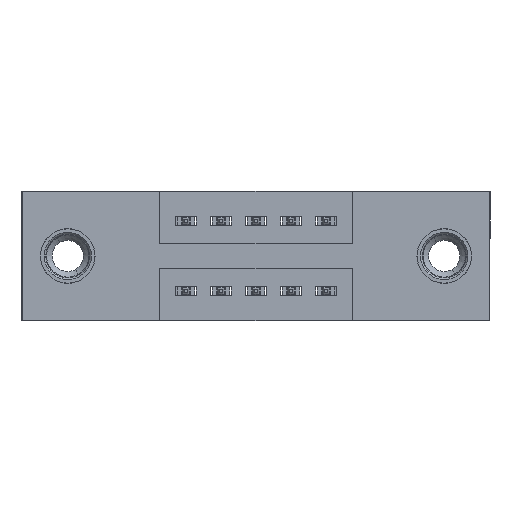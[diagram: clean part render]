
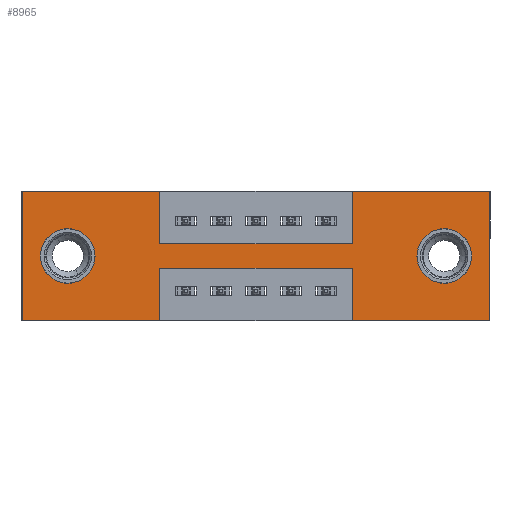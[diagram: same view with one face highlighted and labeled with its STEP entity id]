
A CAD part, front view. The second image highlights one B-rep face of the part: STEP entity #8965.
In plain terms, the highlighted planar face has unit normal (0, -1, 0).
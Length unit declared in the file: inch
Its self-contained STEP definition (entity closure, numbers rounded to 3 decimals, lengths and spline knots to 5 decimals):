
#48 = AXIS2_PLACEMENT_3D ( 'NONE', #10438, #9394, #13650 ) ;
#277 = CARTESIAN_POINT ( 'NONE',  ( 0.3925, 0., -0.15 ) ) ;
#557 = VERTEX_POINT ( 'NONE', #3765 ) ;
#641 = CARTESIAN_POINT ( 'NONE',  ( 0.3925, 0., 0. ) ) ;
#711 = VECTOR ( 'NONE', #12279, 39.37008 ) ;
#821 = EDGE_CURVE ( 'NONE', #13624, #557, #13502, .T. ) ;
#884 = DIRECTION ( 'NONE',  ( 0., 0., 1. ) ) ;
#1006 = CARTESIAN_POINT ( 'NONE',  ( 0.9425, 0., -0.15 ) ) ;
#1064 = VERTEX_POINT ( 'NONE', #1105 ) ;
#1100 = ORIENTED_EDGE ( 'NONE', *, *, #4428, .T. ) ;
#1105 = CARTESIAN_POINT ( 'NONE',  ( 0.3925, 0., 0. ) ) ;
#1164 = ORIENTED_EDGE ( 'NONE', *, *, #11189, .F. ) ;
#1166 = ORIENTED_EDGE ( 'NONE', *, *, #821, .F. ) ;
#1584 = CARTESIAN_POINT ( 'NONE',  ( 1.205, 0., -0.185 ) ) ;
#1680 = EDGE_CURVE ( 'NONE', #5278, #7833, #12041, .T. ) ;
#1694 = EDGE_LOOP ( 'NONE', ( #5590, #1100 ) ) ;
#1700 = LINE ( 'NONE', #2885, #5906 ) ;
#1861 = EDGE_CURVE ( 'NONE', #4488, #11740, #11610, .T. ) ;
#1893 = ORIENTED_EDGE ( 'NONE', *, *, #11238, .F. ) ;
#2094 = CARTESIAN_POINT ( 'NONE',  ( 1.205, 0., -0.107 ) ) ;
#2347 = CARTESIAN_POINT ( 'NONE',  ( 0.3925, 0., -0.37 ) ) ;
#2456 = LINE ( 'NONE', #9901, #4031 ) ;
#2641 = DIRECTION ( 'NONE',  ( 1., 0., 0. ) ) ;
#2816 = ORIENTED_EDGE ( 'NONE', *, *, #5534, .F. ) ;
#2834 = EDGE_CURVE ( 'NONE', #11024, #9593, #13327, .T. ) ;
#2885 = CARTESIAN_POINT ( 'NONE',  ( 1.335, 0., 0. ) ) ;
#3043 = EDGE_LOOP ( 'NONE', ( #2816, #9674, #1893, #11213, #10752, #1164, #8922, #11927, #11122, #3743, #8614, #1166 ) ) ;
#3080 = DIRECTION ( 'NONE',  ( 0., 0., 1. ) ) ;
#3476 = LINE ( 'NONE', #2347, #11236 ) ;
#3632 = EDGE_CURVE ( 'NONE', #11740, #4488, #12515, .T. ) ;
#3658 = VERTEX_POINT ( 'NONE', #11603 ) ;
#3743 = ORIENTED_EDGE ( 'NONE', *, *, #11045, .F. ) ;
#3765 = CARTESIAN_POINT ( 'NONE',  ( 0., 0., -0.37 ) ) ;
#3816 = CARTESIAN_POINT ( 'NONE',  ( 0.3925, 0., -0.22 ) ) ;
#3847 = CARTESIAN_POINT ( 'NONE',  ( 0., 0., -0.37 ) ) ;
#3855 = EDGE_CURVE ( 'NONE', #1064, #4767, #7892, .T. ) ;
#4005 = CARTESIAN_POINT ( 'NONE',  ( 0., 0., 0. ) ) ;
#4031 = VECTOR ( 'NONE', #5877, 39.37008 ) ;
#4333 = LINE ( 'NONE', #12241, #10858 ) ;
#4428 = EDGE_CURVE ( 'NONE', #7833, #5278, #10769, .T. ) ;
#4488 = VERTEX_POINT ( 'NONE', #2094 ) ;
#4767 = VERTEX_POINT ( 'NONE', #277 ) ;
#4917 = DIRECTION ( 'NONE',  ( 0., 0., -1. ) ) ;
#5092 = CARTESIAN_POINT ( 'NONE',  ( 0., 0., -0.37 ) ) ;
#5278 = VERTEX_POINT ( 'NONE', #5466 ) ;
#5466 = CARTESIAN_POINT ( 'NONE',  ( 0.13, 0., -0.107 ) ) ;
#5534 = EDGE_CURVE ( 'NONE', #9593, #13624, #3476, .T. ) ;
#5590 = ORIENTED_EDGE ( 'NONE', *, *, #1680, .T. ) ;
#5665 = LINE ( 'NONE', #6782, #11964 ) ;
#5779 = EDGE_CURVE ( 'NONE', #3658, #8515, #1700, .T. ) ;
#5873 = VERTEX_POINT ( 'NONE', #7197 ) ;
#5877 = DIRECTION ( 'NONE',  ( 1., 0., 0. ) ) ;
#5880 = VECTOR ( 'NONE', #4917, 39.37008 ) ;
#5906 = VECTOR ( 'NONE', #9277, 39.37008 ) ;
#6123 = CARTESIAN_POINT ( 'NONE',  ( 0.9425, 0., 0. ) ) ;
#6212 = FACE_BOUND ( 'NONE', #1694, .T. ) ;
#6420 = VECTOR ( 'NONE', #884, 39.37008 ) ;
#6453 = DIRECTION ( 'NONE',  ( 0., 0., -1. ) ) ;
#6516 = VECTOR ( 'NONE', #10400, 39.37008 ) ;
#6746 = ORIENTED_EDGE ( 'NONE', *, *, #1861, .T. ) ;
#6782 = CARTESIAN_POINT ( 'NONE',  ( 0., 0., 0. ) ) ;
#6832 = LINE ( 'NONE', #13030, #11571 ) ;
#6895 = DIRECTION ( 'NONE',  ( 1., 0., 0. ) ) ;
#6942 = EDGE_CURVE ( 'NONE', #8515, #5873, #8054, .T. ) ;
#7028 = FACE_BOUND ( 'NONE', #9550, .T. ) ;
#7197 = CARTESIAN_POINT ( 'NONE',  ( 0.9425, 0., -0.37 ) ) ;
#7268 = CARTESIAN_POINT ( 'NONE',  ( 0.9425, 0., 0. ) ) ;
#7271 = CARTESIAN_POINT ( 'NONE',  ( 0.13, 0., -0.263 ) ) ;
#7524 = AXIS2_PLACEMENT_3D ( 'NONE', #5092, #10382, #13588 ) ;
#7561 = EDGE_CURVE ( 'NONE', #4767, #9364, #4333, .T. ) ;
#7662 = LINE ( 'NONE', #7923, #11135 ) ;
#7833 = VERTEX_POINT ( 'NONE', #7271 ) ;
#7892 = LINE ( 'NONE', #641, #5880 ) ;
#7923 = CARTESIAN_POINT ( 'NONE',  ( 0., 0., 0. ) ) ;
#8054 = LINE ( 'NONE', #3847, #6516 ) ;
#8146 = EDGE_CURVE ( 'NONE', #557, #9607, #5665, .T. ) ;
#8375 = DIRECTION ( 'NONE',  ( 0., 1., 0. ) ) ;
#8423 = CARTESIAN_POINT ( 'NONE',  ( 1.335, 0., -0.37 ) ) ;
#8515 = VERTEX_POINT ( 'NONE', #8423 ) ;
#8540 = EDGE_CURVE ( 'NONE', #9364, #12619, #10298, .T. ) ;
#8614 = ORIENTED_EDGE ( 'NONE', *, *, #8146, .F. ) ;
#8872 = CARTESIAN_POINT ( 'NONE',  ( 0.3925, 0., -0.37 ) ) ;
#8922 = ORIENTED_EDGE ( 'NONE', *, *, #8540, .F. ) ;
#8965 = ADVANCED_FACE ( 'NONE', ( #7028, #6212, #10317 ), #9268, .T. ) ;
#9268 = PLANE ( 'NONE',  #7524 ) ;
#9277 = DIRECTION ( 'NONE',  ( 0., 0., -1. ) ) ;
#9354 = VECTOR ( 'NONE', #12326, 39.37008 ) ;
#9364 = VERTEX_POINT ( 'NONE', #1006 ) ;
#9394 = DIRECTION ( 'NONE',  ( 0., 1., 0. ) ) ;
#9550 = EDGE_LOOP ( 'NONE', ( #6746, #10355 ) ) ;
#9593 = VERTEX_POINT ( 'NONE', #12086 ) ;
#9607 = VERTEX_POINT ( 'NONE', #4005 ) ;
#9674 = ORIENTED_EDGE ( 'NONE', *, *, #2834, .F. ) ;
#9901 = CARTESIAN_POINT ( 'NONE',  ( 0., 0., 0. ) ) ;
#10147 = DIRECTION ( 'NONE',  ( 0., 0., -1. ) ) ;
#10298 = LINE ( 'NONE', #6123, #6420 ) ;
#10317 = FACE_OUTER_BOUND ( 'NONE', #3043, .T. ) ;
#10355 = ORIENTED_EDGE ( 'NONE', *, *, #3632, .T. ) ;
#10382 = DIRECTION ( 'NONE',  ( 0., -1., 0. ) ) ;
#10400 = DIRECTION ( 'NONE',  ( -1., 0., 0. ) ) ;
#10438 = CARTESIAN_POINT ( 'NONE',  ( 0.13, 0., -0.185 ) ) ;
#10752 = ORIENTED_EDGE ( 'NONE', *, *, #5779, .F. ) ;
#10769 = CIRCLE ( 'NONE', #13239, 0.078 ) ;
#10858 = VECTOR ( 'NONE', #2641, 39.37008 ) ;
#11024 = VERTEX_POINT ( 'NONE', #11991 ) ;
#11045 = EDGE_CURVE ( 'NONE', #9607, #1064, #2456, .T. ) ;
#11122 = ORIENTED_EDGE ( 'NONE', *, *, #3855, .F. ) ;
#11135 = VECTOR ( 'NONE', #6895, 39.37008 ) ;
#11189 = EDGE_CURVE ( 'NONE', #12619, #3658, #7662, .T. ) ;
#11213 = ORIENTED_EDGE ( 'NONE', *, *, #6942, .F. ) ;
#11236 = VECTOR ( 'NONE', #6453, 39.37008 ) ;
#11238 = EDGE_CURVE ( 'NONE', #5873, #11024, #6832, .T. ) ;
#11272 = DIRECTION ( 'NONE',  ( 0., 1., 0. ) ) ;
#11293 = CARTESIAN_POINT ( 'NONE',  ( 0.13, 0., -0.185 ) ) ;
#11422 = CARTESIAN_POINT ( 'NONE',  ( 0., 0., -0.37 ) ) ;
#11571 = VECTOR ( 'NONE', #12966, 39.37008 ) ;
#11603 = CARTESIAN_POINT ( 'NONE',  ( 1.335, 0., 0. ) ) ;
#11610 = CIRCLE ( 'NONE', #12941, 0.078 ) ;
#11638 = AXIS2_PLACEMENT_3D ( 'NONE', #12720, #8375, #12639 ) ;
#11740 = VERTEX_POINT ( 'NONE', #13603 ) ;
#11927 = ORIENTED_EDGE ( 'NONE', *, *, #7561, .F. ) ;
#11964 = VECTOR ( 'NONE', #13316, 39.37008 ) ;
#11991 = CARTESIAN_POINT ( 'NONE',  ( 0.9425, 0., -0.22 ) ) ;
#12041 = CIRCLE ( 'NONE', #48, 0.078 ) ;
#12086 = CARTESIAN_POINT ( 'NONE',  ( 0.3925, 0., -0.22 ) ) ;
#12241 = CARTESIAN_POINT ( 'NONE',  ( 0.3925, 0., -0.15 ) ) ;
#12279 = DIRECTION ( 'NONE',  ( -1., 0., 0. ) ) ;
#12326 = DIRECTION ( 'NONE',  ( -1., 0., 0. ) ) ;
#12515 = CIRCLE ( 'NONE', #11638, 0.078 ) ;
#12606 = DIRECTION ( 'NONE',  ( 0., 1., 0. ) ) ;
#12619 = VERTEX_POINT ( 'NONE', #7268 ) ;
#12639 = DIRECTION ( 'NONE',  ( 0., 0., -1. ) ) ;
#12720 = CARTESIAN_POINT ( 'NONE',  ( 1.205, 0., -0.185 ) ) ;
#12941 = AXIS2_PLACEMENT_3D ( 'NONE', #1584, #11272, #10147 ) ;
#12966 = DIRECTION ( 'NONE',  ( 0., 0., 1. ) ) ;
#13030 = CARTESIAN_POINT ( 'NONE',  ( 0.9425, 0., -0.37 ) ) ;
#13239 = AXIS2_PLACEMENT_3D ( 'NONE', #11293, #12606, #3080 ) ;
#13316 = DIRECTION ( 'NONE',  ( 0., 0., 1. ) ) ;
#13327 = LINE ( 'NONE', #3816, #711 ) ;
#13502 = LINE ( 'NONE', #11422, #9354 ) ;
#13588 = DIRECTION ( 'NONE',  ( 0., 0., -1. ) ) ;
#13603 = CARTESIAN_POINT ( 'NONE',  ( 1.205, 0., -0.263 ) ) ;
#13624 = VERTEX_POINT ( 'NONE', #8872 ) ;
#13650 = DIRECTION ( 'NONE',  ( 0., 0., 1. ) ) ;
